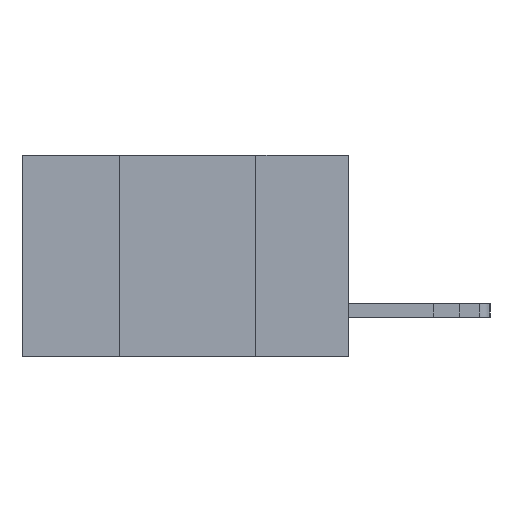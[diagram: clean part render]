
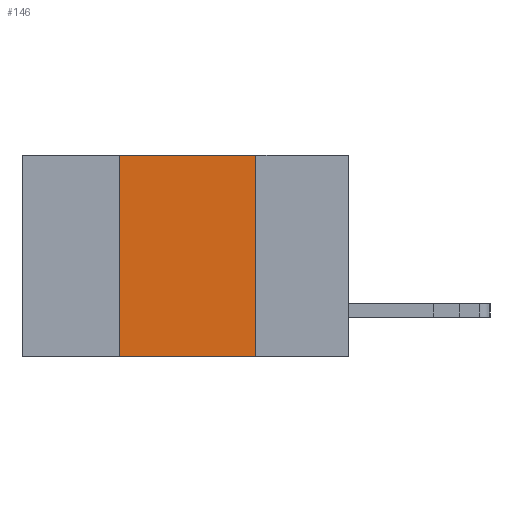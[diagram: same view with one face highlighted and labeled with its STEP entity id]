
A CAD part, left-side view. The second image highlights one B-rep face of the part: STEP entity #146.
In plain terms, the highlighted planar face has unit normal (-1, 0, 0).
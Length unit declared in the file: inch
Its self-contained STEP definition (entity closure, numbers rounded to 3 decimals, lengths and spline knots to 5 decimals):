
#146 = ADVANCED_FACE ( 'NONE', ( #9021 ), #5699, .F. ) ;
#958 = DIRECTION ( 'NONE',  ( 0., -1., 0. ) ) ;
#1314 = CARTESIAN_POINT ( 'NONE',  ( 0., 0.6, -0.37 ) ) ;
#3148 = VECTOR ( 'NONE', #6367, 39.37008 ) ;
#5055 = ORIENTED_EDGE ( 'NONE', *, *, #7038, .T. ) ;
#5478 = VERTEX_POINT ( 'NONE', #20130 ) ;
#5667 = CARTESIAN_POINT ( 'NONE',  ( 0., 0.6, 0. ) ) ;
#5699 = PLANE ( 'NONE',  #15998 ) ;
#5771 = DIRECTION ( 'NONE',  ( 0., 0., -1. ) ) ;
#5918 = VECTOR ( 'NONE', #958, 39.37008 ) ;
#5974 = DIRECTION ( 'NONE',  ( 1., 0., 0. ) ) ;
#6367 = DIRECTION ( 'NONE',  ( 0., 0., 1. ) ) ;
#6512 = CARTESIAN_POINT ( 'NONE',  ( 0., 0.42, 0. ) ) ;
#7038 = EDGE_CURVE ( 'NONE', #13660, #15341, #17290, .T. ) ;
#7119 = CARTESIAN_POINT ( 'NONE',  ( 0., 0.17, 0. ) ) ;
#8083 = LINE ( 'NONE', #16026, #11888 ) ;
#8294 = ORIENTED_EDGE ( 'NONE', *, *, #11771, .F. ) ;
#9021 = FACE_OUTER_BOUND ( 'NONE', #10300, .T. ) ;
#9456 = EDGE_CURVE ( 'NONE', #13660, #16216, #16077, .T. ) ;
#10300 = EDGE_LOOP ( 'NONE', ( #19174, #8294, #17453, #5055 ) ) ;
#11771 = EDGE_CURVE ( 'NONE', #16216, #5478, #8083, .T. ) ;
#11888 = VECTOR ( 'NONE', #12732, 39.37008 ) ;
#12732 = DIRECTION ( 'NONE',  ( 0., -1., 0. ) ) ;
#13613 = DIRECTION ( 'NONE',  ( 0., 0., -1. ) ) ;
#13660 = VERTEX_POINT ( 'NONE', #17838 ) ;
#14750 = CARTESIAN_POINT ( 'NONE',  ( 0., 0.17, -0.37 ) ) ;
#15341 = VERTEX_POINT ( 'NONE', #14750 ) ;
#15998 = AXIS2_PLACEMENT_3D ( 'NONE', #5667, #5974, #5771 ) ;
#16026 = CARTESIAN_POINT ( 'NONE',  ( 0., 0.6, 0. ) ) ;
#16077 = LINE ( 'NONE', #6512, #3148 ) ;
#16216 = VERTEX_POINT ( 'NONE', #20087 ) ;
#16544 = VECTOR ( 'NONE', #13613, 39.37008 ) ;
#17290 = LINE ( 'NONE', #1314, #5918 ) ;
#17453 = ORIENTED_EDGE ( 'NONE', *, *, #9456, .F. ) ;
#17500 = EDGE_CURVE ( 'NONE', #5478, #15341, #20748, .T. ) ;
#17838 = CARTESIAN_POINT ( 'NONE',  ( 0., 0.42, -0.37 ) ) ;
#19174 = ORIENTED_EDGE ( 'NONE', *, *, #17500, .F. ) ;
#20087 = CARTESIAN_POINT ( 'NONE',  ( 0., 0.42, 0. ) ) ;
#20130 = CARTESIAN_POINT ( 'NONE',  ( 0., 0.17, 0. ) ) ;
#20748 = LINE ( 'NONE', #7119, #16544 ) ;
